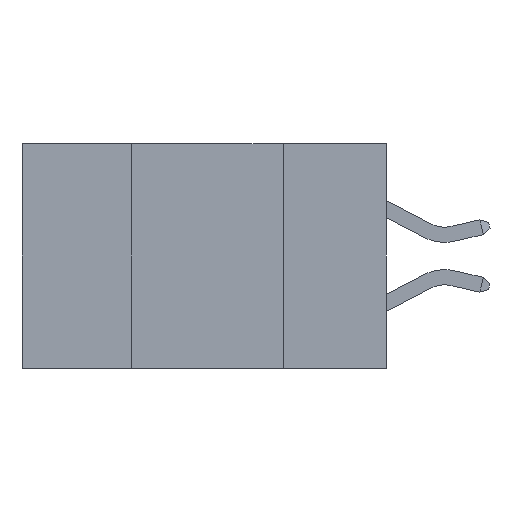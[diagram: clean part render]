
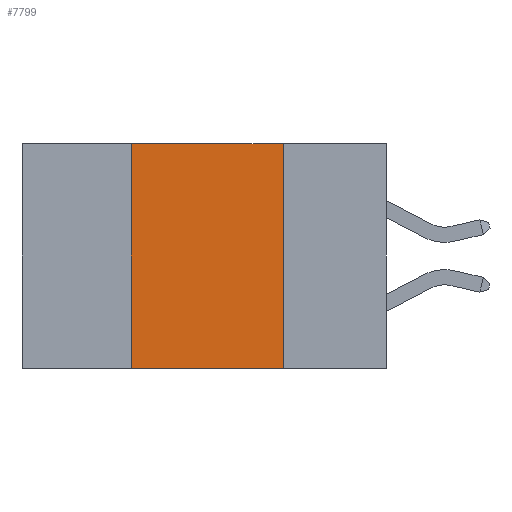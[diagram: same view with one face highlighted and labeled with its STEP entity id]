
A CAD part, left-side view. The second image highlights one B-rep face of the part: STEP entity #7799.
In plain terms, the highlighted planar face has unit normal (-1, 0, 0).
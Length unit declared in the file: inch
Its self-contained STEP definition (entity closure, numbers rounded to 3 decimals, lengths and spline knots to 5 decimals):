
#62 = CARTESIAN_POINT ( 'NONE',  ( 0., 0.6, 0. ) ) ;
#202 = VECTOR ( 'NONE', #11111, 39.37008 ) ;
#470 = VECTOR ( 'NONE', #12041, 39.37008 ) ;
#776 = CARTESIAN_POINT ( 'NONE',  ( 0., 0.6, -0.37 ) ) ;
#882 = EDGE_CURVE ( 'NONE', #4618, #2346, #11948, .T. ) ;
#1162 = DIRECTION ( 'NONE',  ( 0., -1., 0. ) ) ;
#1548 = CARTESIAN_POINT ( 'NONE',  ( 0., 0.42, -0.37 ) ) ;
#1612 = CARTESIAN_POINT ( 'NONE',  ( 0., 0.17, -0.37 ) ) ;
#2142 = LINE ( 'NONE', #776, #12804 ) ;
#2346 = VERTEX_POINT ( 'NONE', #1612 ) ;
#2641 = LINE ( 'NONE', #62, #4758 ) ;
#4395 = ORIENTED_EDGE ( 'NONE', *, *, #4564, .F. ) ;
#4564 = EDGE_CURVE ( 'NONE', #12304, #13118, #9447, .T. ) ;
#4618 = VERTEX_POINT ( 'NONE', #9676 ) ;
#4758 = VECTOR ( 'NONE', #1162, 39.37008 ) ;
#5109 = PLANE ( 'NONE',  #5749 ) ;
#5345 = ORIENTED_EDGE ( 'NONE', *, *, #5754, .T. ) ;
#5749 = AXIS2_PLACEMENT_3D ( 'NONE', #12337, #6145, #13328 ) ;
#5754 = EDGE_CURVE ( 'NONE', #12304, #2346, #2142, .T. ) ;
#5986 = EDGE_CURVE ( 'NONE', #13118, #4618, #2641, .T. ) ;
#6145 = DIRECTION ( 'NONE',  ( 1., 0., 0. ) ) ;
#6558 = EDGE_LOOP ( 'NONE', ( #7280, #8584, #4395, #5345 ) ) ;
#7280 = ORIENTED_EDGE ( 'NONE', *, *, #882, .F. ) ;
#7799 = ADVANCED_FACE ( 'NONE', ( #12546 ), #5109, .F. ) ;
#8218 = CARTESIAN_POINT ( 'NONE',  ( 0., 0.42, 0. ) ) ;
#8584 = ORIENTED_EDGE ( 'NONE', *, *, #5986, .F. ) ;
#9447 = LINE ( 'NONE', #11290, #470 ) ;
#9676 = CARTESIAN_POINT ( 'NONE',  ( 0., 0.17, 0. ) ) ;
#10160 = DIRECTION ( 'NONE',  ( 0., -1., 0. ) ) ;
#11111 = DIRECTION ( 'NONE',  ( 0., 0., -1. ) ) ;
#11290 = CARTESIAN_POINT ( 'NONE',  ( 0., 0.42, 0. ) ) ;
#11948 = LINE ( 'NONE', #12560, #202 ) ;
#12041 = DIRECTION ( 'NONE',  ( 0., 0., 1. ) ) ;
#12304 = VERTEX_POINT ( 'NONE', #1548 ) ;
#12337 = CARTESIAN_POINT ( 'NONE',  ( 0., 0.6, 0. ) ) ;
#12546 = FACE_OUTER_BOUND ( 'NONE', #6558, .T. ) ;
#12560 = CARTESIAN_POINT ( 'NONE',  ( 0., 0.17, 0. ) ) ;
#12804 = VECTOR ( 'NONE', #10160, 39.37008 ) ;
#13118 = VERTEX_POINT ( 'NONE', #8218 ) ;
#13328 = DIRECTION ( 'NONE',  ( 0., 0., -1. ) ) ;
